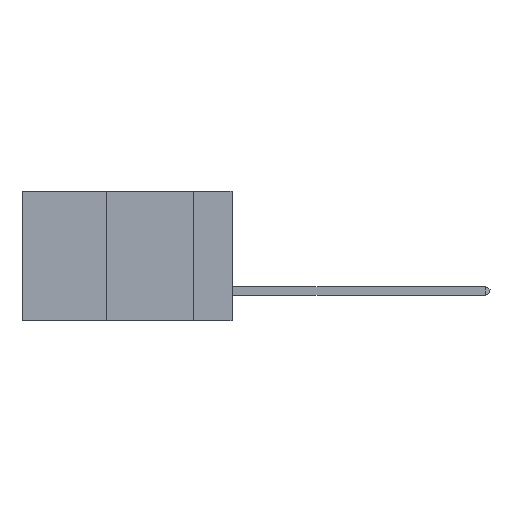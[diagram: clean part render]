
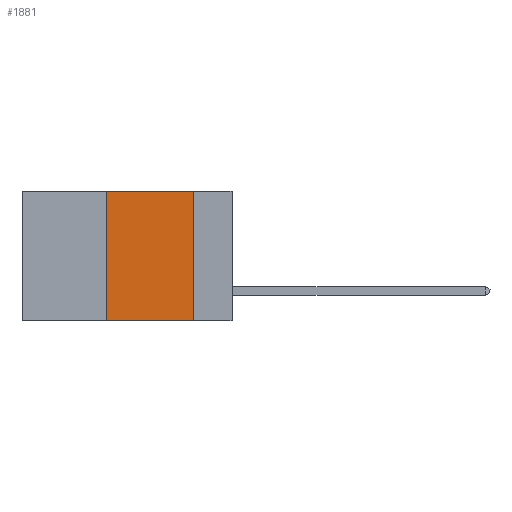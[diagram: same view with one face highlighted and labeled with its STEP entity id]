
A CAD part, left-side view. The second image highlights one B-rep face of the part: STEP entity #1881.
In plain terms, the highlighted planar face has unit normal (-1, 0, 0).
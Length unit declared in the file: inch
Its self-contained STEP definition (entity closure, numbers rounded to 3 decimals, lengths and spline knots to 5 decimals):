
#349 = ORIENTED_EDGE ( 'NONE', *, *, #2914, .F. ) ;
#1172 = LINE ( 'NONE', #3850, #6585 ) ;
#1371 = ORIENTED_EDGE ( 'NONE', *, *, #9397, .F. ) ;
#1410 = LINE ( 'NONE', #9985, #9523 ) ;
#1634 = VERTEX_POINT ( 'NONE', #2667 ) ;
#1881 = ADVANCED_FACE ( 'NONE', ( #7943 ), #9169, .F. ) ;
#2196 = VERTEX_POINT ( 'NONE', #6430 ) ;
#2223 = DIRECTION ( 'NONE',  ( 0., -1., 0. ) ) ;
#2371 = AXIS2_PLACEMENT_3D ( 'NONE', #3791, #4298, #4532 ) ;
#2667 = CARTESIAN_POINT ( 'NONE',  ( 0., 0.11, 0. ) ) ;
#2745 = VECTOR ( 'NONE', #8073, 39.37008 ) ;
#2773 = EDGE_CURVE ( 'NONE', #9814, #2196, #4811, .T. ) ;
#2914 = EDGE_CURVE ( 'NONE', #7186, #1634, #1172, .T. ) ;
#3133 = DIRECTION ( 'NONE',  ( 0., 0., 1. ) ) ;
#3205 = CARTESIAN_POINT ( 'NONE',  ( 0., 0.36, 0. ) ) ;
#3314 = ORIENTED_EDGE ( 'NONE', *, *, #2773, .T. ) ;
#3746 = CARTESIAN_POINT ( 'NONE',  ( 0., 0.36, -0.37 ) ) ;
#3791 = CARTESIAN_POINT ( 'NONE',  ( 0., 0.6, 0. ) ) ;
#3850 = CARTESIAN_POINT ( 'NONE',  ( 0., 0.6, 0. ) ) ;
#4035 = VECTOR ( 'NONE', #3133, 39.37008 ) ;
#4298 = DIRECTION ( 'NONE',  ( 1., 0., 0. ) ) ;
#4416 = CARTESIAN_POINT ( 'NONE',  ( 0., 0.36, 0. ) ) ;
#4532 = DIRECTION ( 'NONE',  ( 0., 0., -1. ) ) ;
#4609 = DIRECTION ( 'NONE',  ( 0., 0., -1. ) ) ;
#4811 = LINE ( 'NONE', #5038, #2745 ) ;
#5038 = CARTESIAN_POINT ( 'NONE',  ( 0., 0.6, -0.37 ) ) ;
#5756 = EDGE_LOOP ( 'NONE', ( #9447, #349, #1371, #3314 ) ) ;
#5849 = EDGE_CURVE ( 'NONE', #1634, #2196, #1410, .T. ) ;
#6430 = CARTESIAN_POINT ( 'NONE',  ( 0., 0.11, -0.37 ) ) ;
#6521 = LINE ( 'NONE', #3205, #4035 ) ;
#6585 = VECTOR ( 'NONE', #2223, 39.37008 ) ;
#7186 = VERTEX_POINT ( 'NONE', #4416 ) ;
#7943 = FACE_OUTER_BOUND ( 'NONE', #5756, .T. ) ;
#8073 = DIRECTION ( 'NONE',  ( 0., -1., 0. ) ) ;
#9169 = PLANE ( 'NONE',  #2371 ) ;
#9397 = EDGE_CURVE ( 'NONE', #9814, #7186, #6521, .T. ) ;
#9447 = ORIENTED_EDGE ( 'NONE', *, *, #5849, .F. ) ;
#9523 = VECTOR ( 'NONE', #4609, 39.37008 ) ;
#9814 = VERTEX_POINT ( 'NONE', #3746 ) ;
#9985 = CARTESIAN_POINT ( 'NONE',  ( 0., 0.11, 0. ) ) ;
